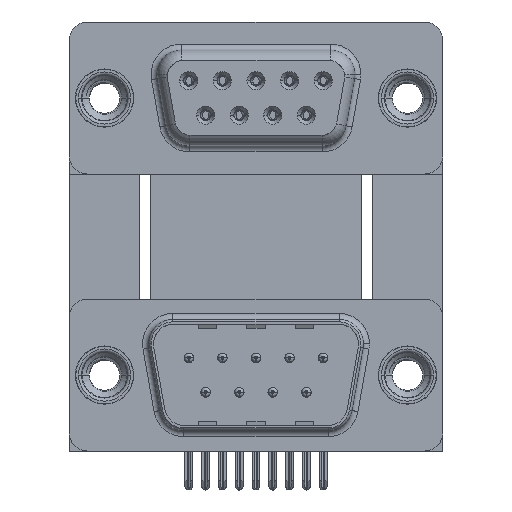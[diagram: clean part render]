
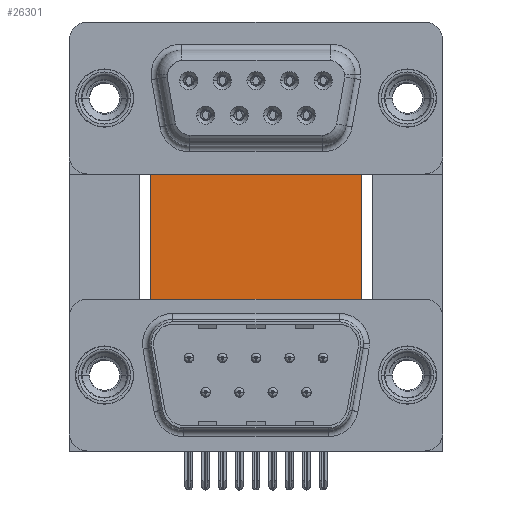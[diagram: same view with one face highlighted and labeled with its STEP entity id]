
A CAD part, top view. The second image highlights one B-rep face of the part: STEP entity #26301.
In plain terms, the highlighted planar face has unit normal (0, 0, 1).
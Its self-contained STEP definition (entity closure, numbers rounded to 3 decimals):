
#234 = ORIENTED_EDGE ( 'NONE', *, *, #7809, .T. ) ;
#472 = AXIS2_PLACEMENT_3D ( 'NONE', #10618, #30778, #7595 ) ;
#707 = ORIENTED_EDGE ( 'NONE', *, *, #25701, .F. ) ;
#1125 = DIRECTION ( 'NONE',  ( 0., 1., 0. ) ) ;
#1269 = DIRECTION ( 'NONE',  ( -0.336, 0.942, 0. ) ) ;
#1662 = ORIENTED_EDGE ( 'NONE', *, *, #14414, .T. ) ;
#2114 = CARTESIAN_POINT ( 'NONE',  ( 2.4, -4.635, -12. ) ) ;
#2182 = ORIENTED_EDGE ( 'NONE', *, *, #17807, .T. ) ;
#2409 = VERTEX_POINT ( 'NONE', #10747 ) ;
#2521 = VECTOR ( 'NONE', #22646, 1000. ) ;
#2773 = LINE ( 'NONE', #34806, #16605 ) ;
#3088 = EDGE_CURVE ( 'NONE', #29152, #2409, #18229, .T. ) ;
#3117 = VECTOR ( 'NONE', #23691, 1000. ) ;
#3263 = CARTESIAN_POINT ( 'NONE',  ( 22.09, -4.635, -12. ) ) ;
#3296 = VERTEX_POINT ( 'NONE', #36854 ) ;
#3498 = CARTESIAN_POINT ( 'NONE',  ( 22.09, -3.735, -12. ) ) ;
#3523 = DIRECTION ( 'NONE',  ( 0., -1., 0. ) ) ;
#3760 = ORIENTED_EDGE ( 'NONE', *, *, #3088, .F. ) ;
#3867 = LINE ( 'NONE', #3498, #14793 ) ;
#3931 = EDGE_CURVE ( 'NONE', #27744, #29813, #21296, .T. ) ;
#4098 = CARTESIAN_POINT ( 'NONE',  ( 22.59, -4.635, -12. ) ) ;
#5220 = VECTOR ( 'NONE', #6955, 1000. ) ;
#5410 = DIRECTION ( 'NONE',  ( 1., 0., 0. ) ) ;
#6874 = DIRECTION ( 'NONE',  ( 0., -1., 0. ) ) ;
#6955 = DIRECTION ( 'NONE',  ( 1., 0., 0. ) ) ;
#7595 = DIRECTION ( 'NONE',  ( -1., 0., 0. ) ) ;
#7809 = EDGE_CURVE ( 'NONE', #22493, #11325, #16568, .T. ) ;
#9648 = CARTESIAN_POINT ( 'NONE',  ( 3.79, -3.735, -12. ) ) ;
#10618 = CARTESIAN_POINT ( 'NONE',  ( 3.79, 16.585, -12. ) ) ;
#10747 = CARTESIAN_POINT ( 'NONE',  ( 21.2, 16.585, -12. ) ) ;
#11325 = VERTEX_POINT ( 'NONE', #16884 ) ;
#11524 = LINE ( 'NONE', #37151, #2521 ) ;
#12266 = CARTESIAN_POINT ( 'NONE',  ( 22.59, -4.635, -12. ) ) ;
#13077 = VECTOR ( 'NONE', #5410, 1000. ) ;
#13379 = ORIENTED_EDGE ( 'NONE', *, *, #14822, .T. ) ;
#13493 = CARTESIAN_POINT ( 'NONE',  ( 3.79, -0.735, -12. ) ) ;
#14414 = EDGE_CURVE ( 'NONE', #29813, #3296, #24068, .T. ) ;
#14793 = VECTOR ( 'NONE', #6874, 1000. ) ;
#14822 = EDGE_CURVE ( 'NONE', #32627, #28375, #30204, .T. ) ;
#15804 = EDGE_CURVE ( 'NONE', #16152, #22493, #11524, .T. ) ;
#16152 = VERTEX_POINT ( 'NONE', #13493 ) ;
#16568 = LINE ( 'NONE', #34057, #13077 ) ;
#16605 = VECTOR ( 'NONE', #31798, 1000. ) ;
#16884 = CARTESIAN_POINT ( 'NONE',  ( 2.9, -4.635, -12. ) ) ;
#17807 = EDGE_CURVE ( 'NONE', #28375, #27744, #3867, .T. ) ;
#17856 = LINE ( 'NONE', #35747, #20193 ) ;
#18229 = LINE ( 'NONE', #24430, #3117 ) ;
#18308 = ORIENTED_EDGE ( 'NONE', *, *, #31169, .T. ) ;
#18354 = ORIENTED_EDGE ( 'NONE', *, *, #15804, .T. ) ;
#20193 = VECTOR ( 'NONE', #3523, 1000. ) ;
#21296 = LINE ( 'NONE', #29770, #5220 ) ;
#22493 = VERTEX_POINT ( 'NONE', #2114 ) ;
#22646 = DIRECTION ( 'NONE',  ( -0.336, -0.942, 0. ) ) ;
#23691 = DIRECTION ( 'NONE',  ( 1., 0., 0. ) ) ;
#24068 = LINE ( 'NONE', #4098, #32052 ) ;
#24430 = CARTESIAN_POINT ( 'NONE',  ( 3.79, 16.585, -12. ) ) ;
#24940 = PLANE ( 'NONE',  #472 ) ;
#25504 = EDGE_CURVE ( 'NONE', #29152, #16152, #2773, .T. ) ;
#25701 = EDGE_CURVE ( 'NONE', #2409, #3296, #17856, .T. ) ;
#26190 = CARTESIAN_POINT ( 'NONE',  ( 22.09, -3.735, -12. ) ) ;
#26301 = ADVANCED_FACE ( 'NONE', ( #36439 ), #24940, .F. ) ;
#26934 = LINE ( 'NONE', #33349, #32028 ) ;
#27372 = DIRECTION ( 'NONE',  ( 1., 0., 0. ) ) ;
#27744 = VERTEX_POINT ( 'NONE', #3263 ) ;
#27853 = CARTESIAN_POINT ( 'NONE',  ( 2.9, -3.735, -12. ) ) ;
#28375 = VERTEX_POINT ( 'NONE', #26190 ) ;
#29152 = VERTEX_POINT ( 'NONE', #33979 ) ;
#29414 = ORIENTED_EDGE ( 'NONE', *, *, #25504, .T. ) ;
#29770 = CARTESIAN_POINT ( 'NONE',  ( 22.09, -4.635, -12. ) ) ;
#29813 = VERTEX_POINT ( 'NONE', #12266 ) ;
#30204 = LINE ( 'NONE', #9648, #33871 ) ;
#30778 = DIRECTION ( 'NONE',  ( 0., 0., -1. ) ) ;
#31169 = EDGE_CURVE ( 'NONE', #11325, #32627, #26934, .T. ) ;
#31631 = ORIENTED_EDGE ( 'NONE', *, *, #3931, .T. ) ;
#31798 = DIRECTION ( 'NONE',  ( 0., -1., 0. ) ) ;
#32028 = VECTOR ( 'NONE', #1125, 1000. ) ;
#32052 = VECTOR ( 'NONE', #1269, 1000. ) ;
#32122 = EDGE_LOOP ( 'NONE', ( #13379, #2182, #31631, #1662, #707, #3760, #29414, #18354, #234, #18308 ) ) ;
#32627 = VERTEX_POINT ( 'NONE', #27853 ) ;
#33349 = CARTESIAN_POINT ( 'NONE',  ( 2.9, -3.735, -12. ) ) ;
#33871 = VECTOR ( 'NONE', #27372, 1000. ) ;
#33979 = CARTESIAN_POINT ( 'NONE',  ( 3.79, 16.585, -12. ) ) ;
#34057 = CARTESIAN_POINT ( 'NONE',  ( 2.9, -4.635, -12. ) ) ;
#34806 = CARTESIAN_POINT ( 'NONE',  ( 3.79, 16.585, -12. ) ) ;
#35747 = CARTESIAN_POINT ( 'NONE',  ( 21.2, 16.585, -12. ) ) ;
#36439 = FACE_OUTER_BOUND ( 'NONE', #32122, .T. ) ;
#36854 = CARTESIAN_POINT ( 'NONE',  ( 21.2, -0.735, -12. ) ) ;
#37151 = CARTESIAN_POINT ( 'NONE',  ( 2.4, -4.635, -12. ) ) ;
